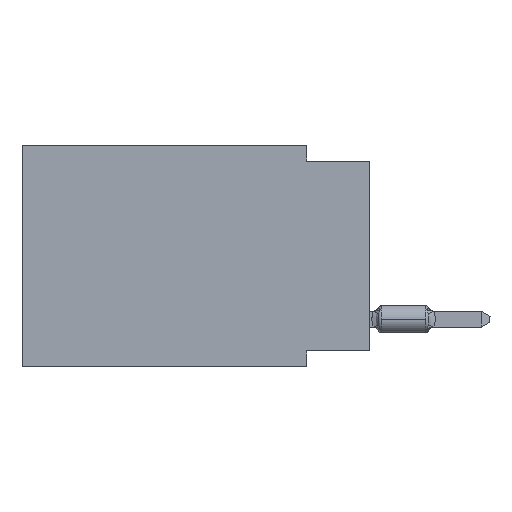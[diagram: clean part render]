
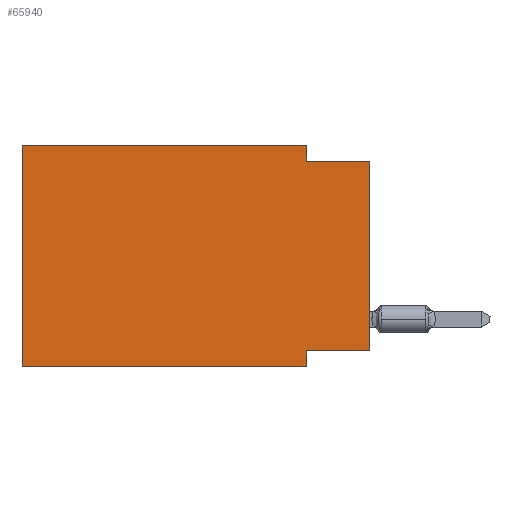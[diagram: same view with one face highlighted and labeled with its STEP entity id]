
A CAD part, left-side view. The second image highlights one B-rep face of the part: STEP entity #65940.
In plain terms, the highlighted planar face has unit normal (-1, 0, 0).
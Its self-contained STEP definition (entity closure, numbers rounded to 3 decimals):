
#1491 = EDGE_CURVE ( 'NONE', #35682, #58295, #96177, .T. ) ;
#3116 = DIRECTION ( 'NONE',  ( 0., 0., -1. ) ) ;
#4643 = ORIENTED_EDGE ( 'NONE', *, *, #31350, .F. ) ;
#6139 = LINE ( 'NONE', #80279, #60869 ) ;
#12884 = CARTESIAN_POINT ( 'NONE',  ( 0., 0., -0.635 ) ) ;
#15918 = CARTESIAN_POINT ( 'NONE',  ( 0., 2.54, 0. ) ) ;
#16493 = ORIENTED_EDGE ( 'NONE', *, *, #93524, .T. ) ;
#16926 = ORIENTED_EDGE ( 'NONE', *, *, #1491, .F. ) ;
#20151 = LINE ( 'NONE', #12884, #41713 ) ;
#22394 = VERTEX_POINT ( 'NONE', #50238 ) ;
#26377 = VECTOR ( 'NONE', #55189, 1000. ) ;
#28159 = EDGE_CURVE ( 'NONE', #22394, #95132, #66038, .T. ) ;
#29882 = ORIENTED_EDGE ( 'NONE', *, *, #51302, .F. ) ;
#30588 = CARTESIAN_POINT ( 'NONE',  ( 0., 13.97, 0. ) ) ;
#31350 = EDGE_CURVE ( 'NONE', #95132, #62384, #20151, .T. ) ;
#32013 = ORIENTED_EDGE ( 'NONE', *, *, #91602, .T. ) ;
#35682 = VERTEX_POINT ( 'NONE', #110028 ) ;
#37158 = VECTOR ( 'NONE', #3116, 1000. ) ;
#37604 = CARTESIAN_POINT ( 'NONE',  ( 0., 13.97, -8.89 ) ) ;
#41713 = VECTOR ( 'NONE', #62470, 1000. ) ;
#43925 = DIRECTION ( 'NONE',  ( 0., -1., 0. ) ) ;
#45254 = ORIENTED_EDGE ( 'NONE', *, *, #28159, .F. ) ;
#46126 = EDGE_CURVE ( 'NONE', #56219, #35682, #89036, .T. ) ;
#46662 = CARTESIAN_POINT ( 'NONE',  ( 0., 0., -8.255 ) ) ;
#47223 = AXIS2_PLACEMENT_3D ( 'NONE', #30588, #89654, #56752 ) ;
#50238 = CARTESIAN_POINT ( 'NONE',  ( 0., 2.54, 0. ) ) ;
#51302 = EDGE_CURVE ( 'NONE', #86561, #103531, #59549, .T. ) ;
#53300 = ORIENTED_EDGE ( 'NONE', *, *, #46126, .F. ) ;
#55189 = DIRECTION ( 'NONE',  ( 0., -1., 0. ) ) ;
#55659 = PLANE ( 'NONE',  #47223 ) ;
#56219 = VERTEX_POINT ( 'NONE', #109154 ) ;
#56752 = DIRECTION ( 'NONE',  ( 0., 0., -1. ) ) ;
#58295 = VERTEX_POINT ( 'NONE', #68327 ) ;
#59549 = LINE ( 'NONE', #93551, #77894 ) ;
#60869 = VECTOR ( 'NONE', #71947, 1000. ) ;
#62384 = VERTEX_POINT ( 'NONE', #104774 ) ;
#62470 = DIRECTION ( 'NONE',  ( 0., -1., 0. ) ) ;
#63321 = VECTOR ( 'NONE', #43925, 1000. ) ;
#64025 = FACE_OUTER_BOUND ( 'NONE', #100680, .T. ) ;
#64645 = LINE ( 'NONE', #107006, #26377 ) ;
#65940 = ADVANCED_FACE ( 'NONE', ( #64025 ), #55659, .F. ) ;
#66038 = LINE ( 'NONE', #15918, #95258 ) ;
#68327 = CARTESIAN_POINT ( 'NONE',  ( 0., 2.54, -8.89 ) ) ;
#70549 = CARTESIAN_POINT ( 'NONE',  ( 0., 2.54, -8.89 ) ) ;
#71947 = DIRECTION ( 'NONE',  ( 0., 0., 1. ) ) ;
#76830 = DIRECTION ( 'NONE',  ( 0., 0., 1. ) ) ;
#77368 = CARTESIAN_POINT ( 'NONE',  ( 0., 13.97, -8.89 ) ) ;
#77894 = VECTOR ( 'NONE', #76830, 1000. ) ;
#80279 = CARTESIAN_POINT ( 'NONE',  ( 0., 0., 0. ) ) ;
#80678 = DIRECTION ( 'NONE',  ( 0., 1., 0. ) ) ;
#80720 = VECTOR ( 'NONE', #80678, 1000. ) ;
#86561 = VERTEX_POINT ( 'NONE', #77368 ) ;
#89036 = LINE ( 'NONE', #46662, #80720 ) ;
#89403 = LINE ( 'NONE', #37604, #63321 ) ;
#89654 = DIRECTION ( 'NONE',  ( 1., 0., 0. ) ) ;
#91602 = EDGE_CURVE ( 'NONE', #86561, #58295, #89403, .T. ) ;
#91637 = CARTESIAN_POINT ( 'NONE',  ( 0., 13.97, 0. ) ) ;
#92369 = CARTESIAN_POINT ( 'NONE',  ( 0., 2.54, -0.635 ) ) ;
#93524 = EDGE_CURVE ( 'NONE', #56219, #62384, #6139, .T. ) ;
#93551 = CARTESIAN_POINT ( 'NONE',  ( 0., 13.97, 0. ) ) ;
#95132 = VERTEX_POINT ( 'NONE', #92369 ) ;
#95258 = VECTOR ( 'NONE', #107315, 1000. ) ;
#96177 = LINE ( 'NONE', #70549, #37158 ) ;
#98717 = ORIENTED_EDGE ( 'NONE', *, *, #100405, .F. ) ;
#100405 = EDGE_CURVE ( 'NONE', #103531, #22394, #64645, .T. ) ;
#100680 = EDGE_LOOP ( 'NONE', ( #16493, #4643, #45254, #98717, #29882, #32013, #16926, #53300 ) ) ;
#103531 = VERTEX_POINT ( 'NONE', #91637 ) ;
#104774 = CARTESIAN_POINT ( 'NONE',  ( 0., 0., -0.635 ) ) ;
#107006 = CARTESIAN_POINT ( 'NONE',  ( 0., 13.97, 0. ) ) ;
#107315 = DIRECTION ( 'NONE',  ( 0., 0., -1. ) ) ;
#109154 = CARTESIAN_POINT ( 'NONE',  ( 0., 0., -8.255 ) ) ;
#110028 = CARTESIAN_POINT ( 'NONE',  ( 0., 2.54, -8.255 ) ) ;
